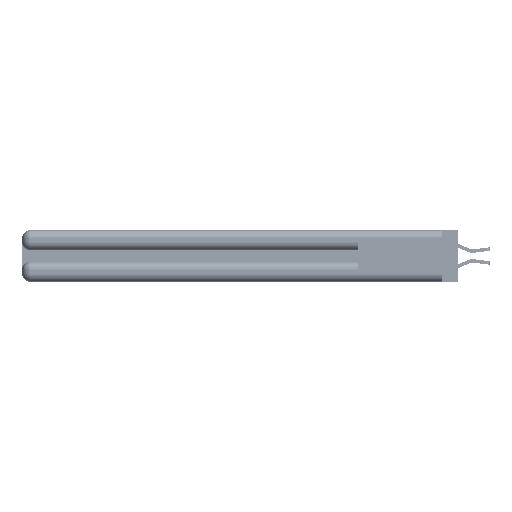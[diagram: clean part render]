
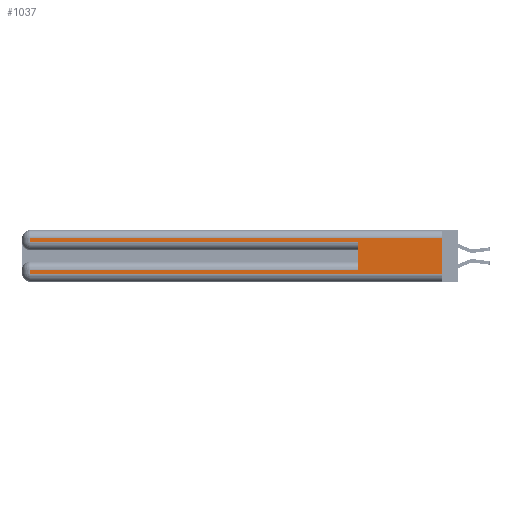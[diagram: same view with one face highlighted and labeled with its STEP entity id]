
A CAD part, left-side view. The second image highlights one B-rep face of the part: STEP entity #1037.
In plain terms, the highlighted planar face has unit normal (-1, 0, 0).
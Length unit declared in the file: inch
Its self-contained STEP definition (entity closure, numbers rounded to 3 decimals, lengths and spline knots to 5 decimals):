
#333 = VERTEX_POINT ( 'NONE', #18016 ) ;
#370 = VECTOR ( 'NONE', #10227, 39.37008 ) ;
#466 = DIRECTION ( 'NONE',  ( 0., 0., 1. ) ) ;
#1037 = ADVANCED_FACE ( 'NONE', ( #7989 ), #18823, .F. ) ;
#1281 = VERTEX_POINT ( 'NONE', #7402 ) ;
#1577 = VECTOR ( 'NONE', #34331, 39.37008 ) ;
#1703 = EDGE_CURVE ( 'NONE', #17475, #333, #18354, .T. ) ;
#2818 = DIRECTION ( 'NONE',  ( 0., 0., -1. ) ) ;
#3155 = VECTOR ( 'NONE', #2818, 39.37008 ) ;
#3605 = LINE ( 'NONE', #17227, #4085 ) ;
#3934 = VECTOR ( 'NONE', #18913, 39.37008 ) ;
#4085 = VECTOR ( 'NONE', #39894, 39.37008 ) ;
#4214 = VECTOR ( 'NONE', #40647, 39.37008 ) ;
#5839 = CARTESIAN_POINT ( 'NONE',  ( 0., 0., 0.37 ) ) ;
#7327 = VERTEX_POINT ( 'NONE', #9185 ) ;
#7402 = CARTESIAN_POINT ( 'NONE',  ( 0., 2.94, 0.285 ) ) ;
#7989 = FACE_OUTER_BOUND ( 'NONE', #13548, .T. ) ;
#9185 = CARTESIAN_POINT ( 'NONE',  ( 0., 2.94, 0.06 ) ) ;
#9838 = ORIENTED_EDGE ( 'NONE', *, *, #12382, .T. ) ;
#9957 = LINE ( 'NONE', #38956, #370 ) ;
#10227 = DIRECTION ( 'NONE',  ( 0., 0., -1. ) ) ;
#12382 = EDGE_CURVE ( 'NONE', #333, #7327, #31469, .T. ) ;
#12879 = CARTESIAN_POINT ( 'NONE',  ( 0., 0., 0.31 ) ) ;
#12889 = EDGE_CURVE ( 'NONE', #13991, #1281, #16748, .T. ) ;
#13548 = EDGE_LOOP ( 'NONE', ( #40329, #31704, #38238, #28720, #17714, #15688, #9838, #30631 ) ) ;
#13991 = VERTEX_POINT ( 'NONE', #28276 ) ;
#14263 = CARTESIAN_POINT ( 'NONE',  ( 0., 0., 0.06 ) ) ;
#15688 = ORIENTED_EDGE ( 'NONE', *, *, #1703, .T. ) ;
#16726 = DIRECTION ( 'NONE',  ( 0., 0., -1. ) ) ;
#16748 = LINE ( 'NONE', #35461, #27904 ) ;
#17104 = VERTEX_POINT ( 'NONE', #21528 ) ;
#17227 = CARTESIAN_POINT ( 'NONE',  ( 0., 0., 0.285 ) ) ;
#17475 = VERTEX_POINT ( 'NONE', #23627 ) ;
#17714 = ORIENTED_EDGE ( 'NONE', *, *, #26256, .F. ) ;
#18016 = CARTESIAN_POINT ( 'NONE',  ( 0., 2.94, 0.085 ) ) ;
#18354 = LINE ( 'NONE', #27627, #4214 ) ;
#18823 = PLANE ( 'NONE',  #27022 ) ;
#18913 = DIRECTION ( 'NONE',  ( 0., 1., 0. ) ) ;
#20755 = EDGE_CURVE ( 'NONE', #1281, #17104, #3605, .T. ) ;
#21528 = CARTESIAN_POINT ( 'NONE',  ( 0., 0.6, 0.285 ) ) ;
#21835 = LINE ( 'NONE', #34459, #1577 ) ;
#21958 = DIRECTION ( 'NONE',  ( 0., 0., -1. ) ) ;
#22319 = CARTESIAN_POINT ( 'NONE',  ( 0., 2.94, 0.37 ) ) ;
#22848 = VECTOR ( 'NONE', #466, 39.37008 ) ;
#23627 = CARTESIAN_POINT ( 'NONE',  ( 0., 0.6, 0.085 ) ) ;
#26256 = EDGE_CURVE ( 'NONE', #17475, #17104, #30952, .T. ) ;
#27022 = AXIS2_PLACEMENT_3D ( 'NONE', #5839, #38077, #21958 ) ;
#27627 = CARTESIAN_POINT ( 'NONE',  ( 0., 0., 0.085 ) ) ;
#27904 = VECTOR ( 'NONE', #16726, 39.37008 ) ;
#28261 = EDGE_CURVE ( 'NONE', #41473, #13991, #40377, .T. ) ;
#28276 = CARTESIAN_POINT ( 'NONE',  ( 0., 2.94, 0.31 ) ) ;
#28720 = ORIENTED_EDGE ( 'NONE', *, *, #20755, .T. ) ;
#30631 = ORIENTED_EDGE ( 'NONE', *, *, #32172, .T. ) ;
#30952 = LINE ( 'NONE', #36214, #22848 ) ;
#31469 = LINE ( 'NONE', #22319, #3155 ) ;
#31704 = ORIENTED_EDGE ( 'NONE', *, *, #28261, .T. ) ;
#32172 = EDGE_CURVE ( 'NONE', #7327, #33156, #21835, .T. ) ;
#33156 = VERTEX_POINT ( 'NONE', #14263 ) ;
#34331 = DIRECTION ( 'NONE',  ( 0., -1., 0. ) ) ;
#34459 = CARTESIAN_POINT ( 'NONE',  ( 0., 0., 0.06 ) ) ;
#35461 = CARTESIAN_POINT ( 'NONE',  ( 0., 2.94, 0.37 ) ) ;
#35721 = EDGE_CURVE ( 'NONE', #41473, #33156, #9957, .T. ) ;
#36214 = CARTESIAN_POINT ( 'NONE',  ( 0., 0.6, 0.145 ) ) ;
#38077 = DIRECTION ( 'NONE',  ( 1., 0., 0. ) ) ;
#38238 = ORIENTED_EDGE ( 'NONE', *, *, #12889, .T. ) ;
#38296 = CARTESIAN_POINT ( 'NONE',  ( 0., 0., 0.31 ) ) ;
#38956 = CARTESIAN_POINT ( 'NONE',  ( 0., 0., 0.37 ) ) ;
#39894 = DIRECTION ( 'NONE',  ( 0., -1., 0. ) ) ;
#40329 = ORIENTED_EDGE ( 'NONE', *, *, #35721, .F. ) ;
#40377 = LINE ( 'NONE', #38296, #3934 ) ;
#40647 = DIRECTION ( 'NONE',  ( 0., 1., 0. ) ) ;
#41473 = VERTEX_POINT ( 'NONE', #12879 ) ;
